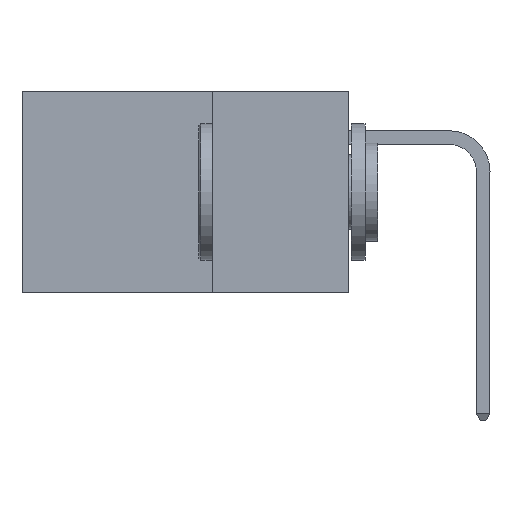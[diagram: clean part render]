
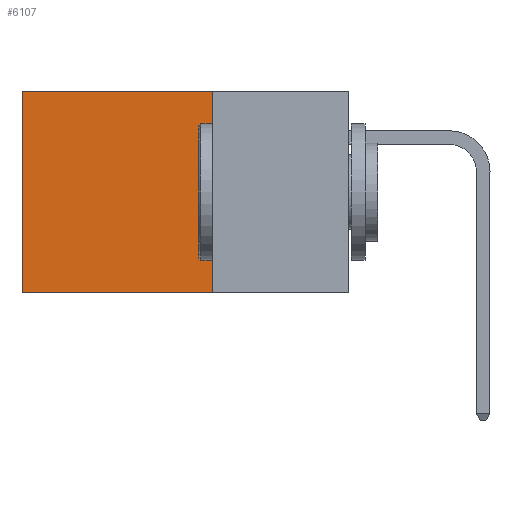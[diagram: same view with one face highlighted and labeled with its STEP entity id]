
A CAD part, left-side view. The second image highlights one B-rep face of the part: STEP entity #6107.
In plain terms, the highlighted planar face has unit normal (-1, 0, 0).
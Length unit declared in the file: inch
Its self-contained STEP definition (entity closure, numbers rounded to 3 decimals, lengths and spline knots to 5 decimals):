
#343 = CARTESIAN_POINT ( 'NONE',  ( 0.2875, 0.6, 0. ) ) ;
#706 = VECTOR ( 'NONE', #5070, 39.37008 ) ;
#731 = FACE_OUTER_BOUND ( 'NONE', #1550, .T. ) ;
#1411 = EDGE_CURVE ( 'NONE', #6194, #2721, #7350, .T. ) ;
#1550 = EDGE_LOOP ( 'NONE', ( #8802, #4804, #2080, #2418 ) ) ;
#1654 = EDGE_CURVE ( 'NONE', #7477, #2721, #5048, .T. ) ;
#1718 = DIRECTION ( 'NONE',  ( 0., 0., -1. ) ) ;
#1870 = VECTOR ( 'NONE', #8632, 39.37008 ) ;
#1907 = AXIS2_PLACEMENT_3D ( 'NONE', #2509, #4745, #5476 ) ;
#2080 = ORIENTED_EDGE ( 'NONE', *, *, #4814, .F. ) ;
#2418 = ORIENTED_EDGE ( 'NONE', *, *, #7452, .T. ) ;
#2509 = CARTESIAN_POINT ( 'NONE',  ( 0.2875, 0.25, 0. ) ) ;
#2721 = VERTEX_POINT ( 'NONE', #5771 ) ;
#2842 = CARTESIAN_POINT ( 'NONE',  ( 0.2875, 0.25, 0. ) ) ;
#2931 = LINE ( 'NONE', #6073, #8903 ) ;
#3572 = VECTOR ( 'NONE', #6909, 39.37008 ) ;
#4024 = LINE ( 'NONE', #2842, #1870 ) ;
#4745 = DIRECTION ( 'NONE',  ( 1., 0., 0. ) ) ;
#4804 = ORIENTED_EDGE ( 'NONE', *, *, #1411, .F. ) ;
#4814 = EDGE_CURVE ( 'NONE', #7413, #6194, #2931, .T. ) ;
#4964 = CARTESIAN_POINT ( 'NONE',  ( 0.2875, 0.6, 0. ) ) ;
#5048 = LINE ( 'NONE', #343, #3572 ) ;
#5070 = DIRECTION ( 'NONE',  ( 0., 1., 0. ) ) ;
#5476 = DIRECTION ( 'NONE',  ( 0., 0., -1. ) ) ;
#5771 = CARTESIAN_POINT ( 'NONE',  ( 0.2875, 0.6, -0.37 ) ) ;
#6073 = CARTESIAN_POINT ( 'NONE',  ( 0.2875, 0.25, 0. ) ) ;
#6107 = ADVANCED_FACE ( 'NONE', ( #731 ), #8516, .F. ) ;
#6194 = VERTEX_POINT ( 'NONE', #7183 ) ;
#6909 = DIRECTION ( 'NONE',  ( 0., 0., -1. ) ) ;
#7131 = CARTESIAN_POINT ( 'NONE',  ( 0.2875, 0.25, 0. ) ) ;
#7183 = CARTESIAN_POINT ( 'NONE',  ( 0.2875, 0.25, -0.37 ) ) ;
#7211 = CARTESIAN_POINT ( 'NONE',  ( 0.2875, 0.25, -0.37 ) ) ;
#7350 = LINE ( 'NONE', #7211, #706 ) ;
#7413 = VERTEX_POINT ( 'NONE', #7131 ) ;
#7452 = EDGE_CURVE ( 'NONE', #7413, #7477, #4024, .T. ) ;
#7477 = VERTEX_POINT ( 'NONE', #4964 ) ;
#8516 = PLANE ( 'NONE',  #1907 ) ;
#8632 = DIRECTION ( 'NONE',  ( 0., 1., 0. ) ) ;
#8802 = ORIENTED_EDGE ( 'NONE', *, *, #1654, .T. ) ;
#8903 = VECTOR ( 'NONE', #1718, 39.37008 ) ;
